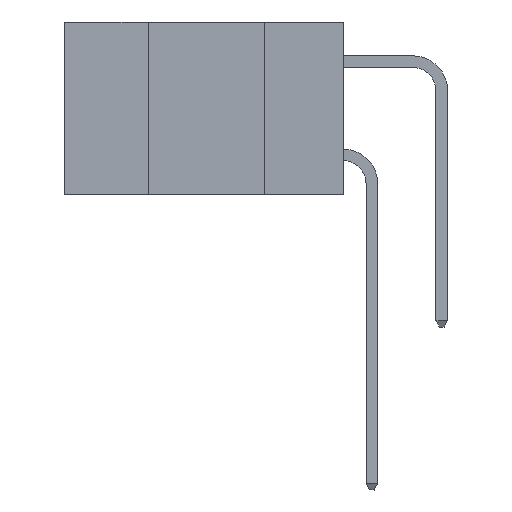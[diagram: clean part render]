
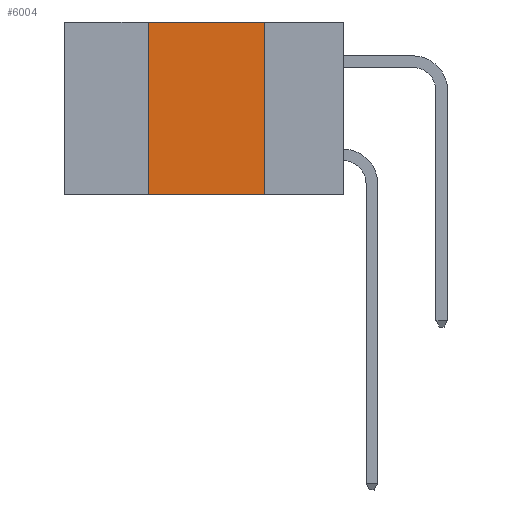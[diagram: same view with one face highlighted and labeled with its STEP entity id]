
A CAD part, left-side view. The second image highlights one B-rep face of the part: STEP entity #6004.
In plain terms, the highlighted planar face has unit normal (-1, 0, 0).
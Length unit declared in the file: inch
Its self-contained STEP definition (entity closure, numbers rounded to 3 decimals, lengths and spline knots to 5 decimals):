
#74 = CARTESIAN_POINT ( 'NONE',  ( 0., 0.42, 0. ) ) ;
#111 = EDGE_CURVE ( 'NONE', #7599, #8520, #12458, .T. ) ;
#352 = CARTESIAN_POINT ( 'NONE',  ( 0., 0.6, 0. ) ) ;
#420 = DIRECTION ( 'NONE',  ( 0., 0., -1. ) ) ;
#641 = EDGE_CURVE ( 'NONE', #8520, #11769, #9165, .T. ) ;
#1078 = CARTESIAN_POINT ( 'NONE',  ( 0., 0.6, -0.37 ) ) ;
#1138 = VECTOR ( 'NONE', #5415, 39.37008 ) ;
#2798 = CARTESIAN_POINT ( 'NONE',  ( 0., 0.17, 0. ) ) ;
#3077 = AXIS2_PLACEMENT_3D ( 'NONE', #352, #7874, #420 ) ;
#4626 = FACE_OUTER_BOUND ( 'NONE', #11091, .T. ) ;
#4659 = DIRECTION ( 'NONE',  ( 0., 0., 1. ) ) ;
#5135 = VERTEX_POINT ( 'NONE', #10787 ) ;
#5415 = DIRECTION ( 'NONE',  ( 0., -1., 0. ) ) ;
#5715 = CARTESIAN_POINT ( 'NONE',  ( 0., 0.17, -0.37 ) ) ;
#6004 = ADVANCED_FACE ( 'NONE', ( #4626 ), #10995, .F. ) ;
#6714 = ORIENTED_EDGE ( 'NONE', *, *, #6988, .F. ) ;
#6977 = CARTESIAN_POINT ( 'NONE',  ( 0., 0.6, 0. ) ) ;
#6988 = EDGE_CURVE ( 'NONE', #5135, #7599, #7908, .T. ) ;
#7172 = ORIENTED_EDGE ( 'NONE', *, *, #641, .F. ) ;
#7599 = VERTEX_POINT ( 'NONE', #74 ) ;
#7874 = DIRECTION ( 'NONE',  ( 1., 0., 0. ) ) ;
#7908 = LINE ( 'NONE', #7979, #13099 ) ;
#7979 = CARTESIAN_POINT ( 'NONE',  ( 0., 0.42, -0.37 ) ) ;
#8520 = VERTEX_POINT ( 'NONE', #2798 ) ;
#8741 = LINE ( 'NONE', #1078, #1138 ) ;
#9165 = LINE ( 'NONE', #5715, #12896 ) ;
#9224 = DIRECTION ( 'NONE',  ( 0., -1., 0. ) ) ;
#10581 = VECTOR ( 'NONE', #9224, 39.37008 ) ;
#10787 = CARTESIAN_POINT ( 'NONE',  ( 0., 0.42, -0.37 ) ) ;
#10995 = PLANE ( 'NONE',  #3077 ) ;
#11017 = ORIENTED_EDGE ( 'NONE', *, *, #12260, .T. ) ;
#11091 = EDGE_LOOP ( 'NONE', ( #7172, #13616, #6714, #11017 ) ) ;
#11322 = DIRECTION ( 'NONE',  ( 0., 0., -1. ) ) ;
#11769 = VERTEX_POINT ( 'NONE', #13767 ) ;
#12260 = EDGE_CURVE ( 'NONE', #5135, #11769, #8741, .T. ) ;
#12458 = LINE ( 'NONE', #6977, #10581 ) ;
#12896 = VECTOR ( 'NONE', #11322, 39.37008 ) ;
#13099 = VECTOR ( 'NONE', #4659, 39.37008 ) ;
#13616 = ORIENTED_EDGE ( 'NONE', *, *, #111, .F. ) ;
#13767 = CARTESIAN_POINT ( 'NONE',  ( 0., 0.17, -0.37 ) ) ;
